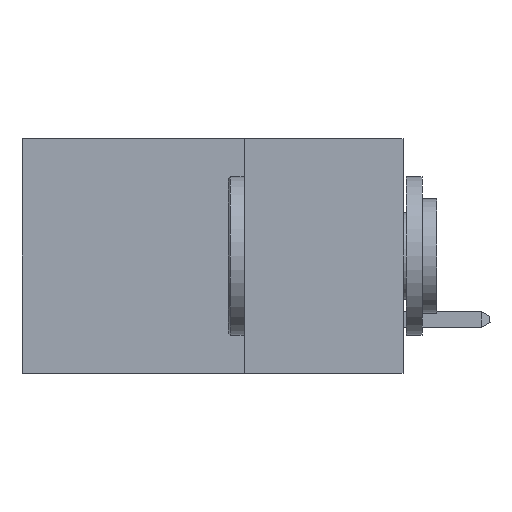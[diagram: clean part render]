
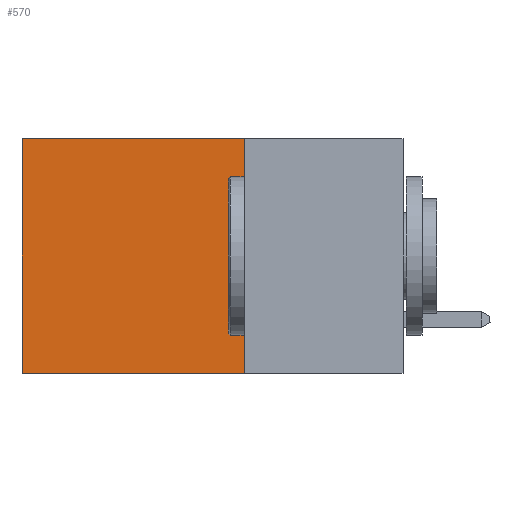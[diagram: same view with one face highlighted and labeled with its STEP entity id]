
A CAD part, left-side view. The second image highlights one B-rep face of the part: STEP entity #570.
In plain terms, the highlighted planar face has unit normal (-1, 0, 0).
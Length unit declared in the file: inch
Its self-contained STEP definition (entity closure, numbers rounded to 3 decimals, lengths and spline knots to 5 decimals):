
#570 = ADVANCED_FACE ( 'NONE', ( #20352 ), #2976, .F. ) ;
#1458 = CARTESIAN_POINT ( 'NONE',  ( 0.2875, 0.6, 0. ) ) ;
#2218 = CARTESIAN_POINT ( 'NONE',  ( 0.2875, 0.25, 0. ) ) ;
#2461 = CARTESIAN_POINT ( 'NONE',  ( 0.2875, 0.6, -0.37 ) ) ;
#2894 = DIRECTION ( 'NONE',  ( 0., 0., -1. ) ) ;
#2970 = DIRECTION ( 'NONE',  ( 1., 0., 0. ) ) ;
#2976 = PLANE ( 'NONE',  #7017 ) ;
#3016 = VERTEX_POINT ( 'NONE', #1458 ) ;
#4138 = LINE ( 'NONE', #14725, #13875 ) ;
#5164 = VECTOR ( 'NONE', #12073, 39.37008 ) ;
#6521 = ORIENTED_EDGE ( 'NONE', *, *, #20115, .T. ) ;
#6608 = VERTEX_POINT ( 'NONE', #10680 ) ;
#7017 = AXIS2_PLACEMENT_3D ( 'NONE', #2218, #2970, #2894 ) ;
#7073 = VERTEX_POINT ( 'NONE', #23357 ) ;
#8077 = LINE ( 'NONE', #18312, #17631 ) ;
#8813 = DIRECTION ( 'NONE',  ( 0., 0., -1. ) ) ;
#9206 = EDGE_CURVE ( 'NONE', #3016, #21846, #4138, .T. ) ;
#9375 = CARTESIAN_POINT ( 'NONE',  ( 0.2875, 0.25, 0. ) ) ;
#9847 = LINE ( 'NONE', #23336, #5164 ) ;
#10680 = CARTESIAN_POINT ( 'NONE',  ( 0.2875, 0.25, 0. ) ) ;
#11079 = DIRECTION ( 'NONE',  ( 0., 0., -1. ) ) ;
#12073 = DIRECTION ( 'NONE',  ( 0., 1., 0. ) ) ;
#13309 = EDGE_LOOP ( 'NONE', ( #19542, #16146, #19923, #6521 ) ) ;
#13875 = VECTOR ( 'NONE', #11079, 39.37008 ) ;
#14725 = CARTESIAN_POINT ( 'NONE',  ( 0.2875, 0.6, 0. ) ) ;
#16146 = ORIENTED_EDGE ( 'NONE', *, *, #22364, .F. ) ;
#17367 = EDGE_CURVE ( 'NONE', #6608, #7073, #8077, .T. ) ;
#17631 = VECTOR ( 'NONE', #8813, 39.37008 ) ;
#18312 = CARTESIAN_POINT ( 'NONE',  ( 0.2875, 0.25, 0. ) ) ;
#19542 = ORIENTED_EDGE ( 'NONE', *, *, #9206, .T. ) ;
#19923 = ORIENTED_EDGE ( 'NONE', *, *, #17367, .F. ) ;
#20115 = EDGE_CURVE ( 'NONE', #6608, #3016, #23734, .T. ) ;
#20352 = FACE_OUTER_BOUND ( 'NONE', #13309, .T. ) ;
#21846 = VERTEX_POINT ( 'NONE', #2461 ) ;
#22364 = EDGE_CURVE ( 'NONE', #7073, #21846, #9847, .T. ) ;
#22548 = DIRECTION ( 'NONE',  ( 0., 1., 0. ) ) ;
#23169 = VECTOR ( 'NONE', #22548, 39.37008 ) ;
#23336 = CARTESIAN_POINT ( 'NONE',  ( 0.2875, 0.25, -0.37 ) ) ;
#23357 = CARTESIAN_POINT ( 'NONE',  ( 0.2875, 0.25, -0.37 ) ) ;
#23734 = LINE ( 'NONE', #9375, #23169 ) ;
